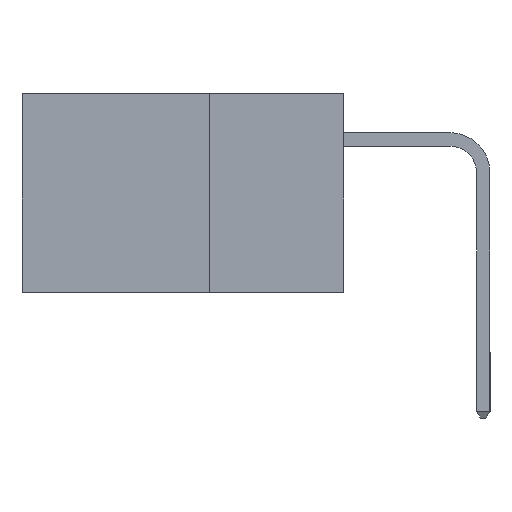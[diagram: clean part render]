
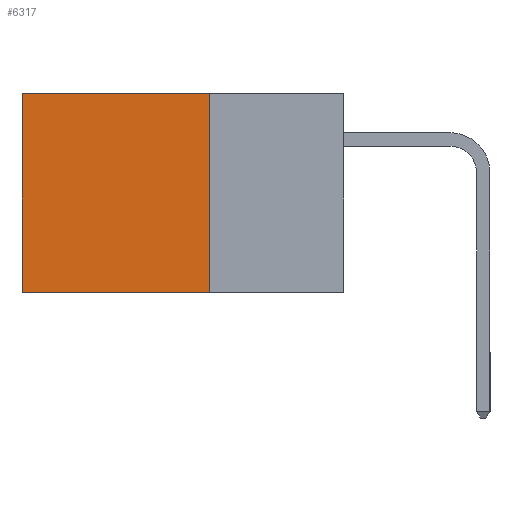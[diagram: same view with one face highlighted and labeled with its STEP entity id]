
A CAD part, left-side view. The second image highlights one B-rep face of the part: STEP entity #6317.
In plain terms, the highlighted planar face has unit normal (-1, 0, 0).
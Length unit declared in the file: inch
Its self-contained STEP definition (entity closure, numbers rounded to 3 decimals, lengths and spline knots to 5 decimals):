
#288 = FACE_OUTER_BOUND ( 'NONE', #947, .T. ) ;
#947 = EDGE_LOOP ( 'NONE', ( #12515, #9425, #18428, #15378 ) ) ;
#3535 = CARTESIAN_POINT ( 'NONE',  ( 0.2615, 0.25, -0.37 ) ) ;
#3903 = VERTEX_POINT ( 'NONE', #20514 ) ;
#4028 = DIRECTION ( 'NONE',  ( 0., 0., -1. ) ) ;
#4039 = VECTOR ( 'NONE', #20762, 39.37008 ) ;
#4835 = EDGE_CURVE ( 'NONE', #7902, #3903, #22737, .T. ) ;
#6317 = ADVANCED_FACE ( 'NONE', ( #288 ), #18511, .F. ) ;
#6916 = DIRECTION ( 'NONE',  ( 0., 0., -1. ) ) ;
#7034 = LINE ( 'NONE', #3535, #9968 ) ;
#7316 = VERTEX_POINT ( 'NONE', #15048 ) ;
#7643 = EDGE_CURVE ( 'NONE', #7316, #11993, #11706, .T. ) ;
#7902 = VERTEX_POINT ( 'NONE', #8691 ) ;
#8691 = CARTESIAN_POINT ( 'NONE',  ( 0.2615, 0.25, -0.37 ) ) ;
#9359 = EDGE_CURVE ( 'NONE', #11993, #3903, #20183, .T. ) ;
#9425 = ORIENTED_EDGE ( 'NONE', *, *, #4835, .F. ) ;
#9436 = CARTESIAN_POINT ( 'NONE',  ( 0.2615, 0.25, 0. ) ) ;
#9968 = VECTOR ( 'NONE', #6916, 39.37008 ) ;
#11696 = VECTOR ( 'NONE', #20926, 39.37008 ) ;
#11706 = LINE ( 'NONE', #9436, #4039 ) ;
#11993 = VERTEX_POINT ( 'NONE', #12905 ) ;
#12515 = ORIENTED_EDGE ( 'NONE', *, *, #9359, .T. ) ;
#12905 = CARTESIAN_POINT ( 'NONE',  ( 0.2615, 0.6, 0. ) ) ;
#13568 = CARTESIAN_POINT ( 'NONE',  ( 0.2615, 0.25, -0.37 ) ) ;
#14545 = EDGE_CURVE ( 'NONE', #7316, #7902, #7034, .T. ) ;
#15048 = CARTESIAN_POINT ( 'NONE',  ( 0.2615, 0.25, 0. ) ) ;
#15378 = ORIENTED_EDGE ( 'NONE', *, *, #7643, .T. ) ;
#16707 = CARTESIAN_POINT ( 'NONE',  ( 0.2615, 0.25, -0.37 ) ) ;
#16831 = DIRECTION ( 'NONE',  ( 1., 0., 0. ) ) ;
#17172 = VECTOR ( 'NONE', #22352, 39.37008 ) ;
#18377 = CARTESIAN_POINT ( 'NONE',  ( 0.2615, 0.6, -0.37 ) ) ;
#18428 = ORIENTED_EDGE ( 'NONE', *, *, #14545, .F. ) ;
#18511 = PLANE ( 'NONE',  #21399 ) ;
#20183 = LINE ( 'NONE', #18377, #17172 ) ;
#20514 = CARTESIAN_POINT ( 'NONE',  ( 0.2615, 0.6, -0.37 ) ) ;
#20762 = DIRECTION ( 'NONE',  ( 0., 1., 0. ) ) ;
#20926 = DIRECTION ( 'NONE',  ( 0., 1., 0. ) ) ;
#21399 = AXIS2_PLACEMENT_3D ( 'NONE', #16707, #16831, #4028 ) ;
#22352 = DIRECTION ( 'NONE',  ( 0., 0., -1. ) ) ;
#22737 = LINE ( 'NONE', #13568, #11696 ) ;
